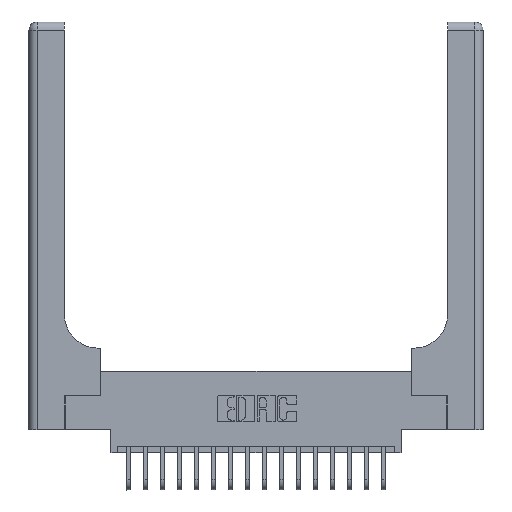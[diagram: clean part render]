
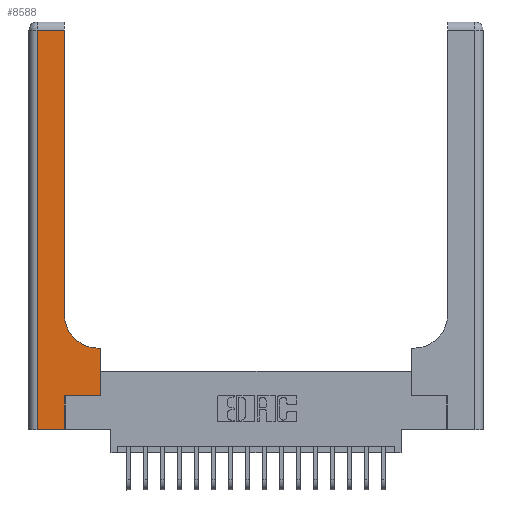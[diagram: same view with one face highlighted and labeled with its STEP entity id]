
A CAD part, top view. The second image highlights one B-rep face of the part: STEP entity #8588.
In plain terms, the highlighted planar face has unit normal (0, 0, 1).
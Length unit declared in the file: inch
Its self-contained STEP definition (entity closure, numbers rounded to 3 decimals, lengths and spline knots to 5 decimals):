
#76 = DIRECTION ( 'NONE',  ( 1., 0., 0. ) ) ;
#202 = EDGE_LOOP ( 'NONE', ( #3198, #1127, #1689, #18911, #7406, #10585, #1963, #21030, #20210 ) ) ;
#544 = VERTEX_POINT ( 'NONE', #6140 ) ;
#554 = DIRECTION ( 'NONE',  ( 1., 0., 0. ) ) ;
#799 = FACE_OUTER_BOUND ( 'NONE', #202, .T. ) ;
#1127 = ORIENTED_EDGE ( 'NONE', *, *, #20029, .T. ) ;
#1205 = AXIS2_PLACEMENT_3D ( 'NONE', #17898, #9666, #76 ) ;
#1557 = VECTOR ( 'NONE', #20072, 39.37008 ) ;
#1689 = ORIENTED_EDGE ( 'NONE', *, *, #18613, .T. ) ;
#1963 = ORIENTED_EDGE ( 'NONE', *, *, #7899, .T. ) ;
#1978 = LINE ( 'NONE', #5490, #5737 ) ;
#2013 = LINE ( 'NONE', #16639, #17235 ) ;
#2168 = CARTESIAN_POINT ( 'NONE',  ( 0.06, 3., 0.37 ) ) ;
#2465 = VERTEX_POINT ( 'NONE', #7567 ) ;
#2975 = EDGE_CURVE ( 'NONE', #14000, #4491, #12141, .T. ) ;
#3198 = ORIENTED_EDGE ( 'NONE', *, *, #15015, .T. ) ;
#3808 = DIRECTION ( 'NONE',  ( 0., 0., -1. ) ) ;
#4002 = CARTESIAN_POINT ( 'NONE',  ( 0.265, 0.25, 0.37 ) ) ;
#4491 = VERTEX_POINT ( 'NONE', #15877 ) ;
#4868 = CARTESIAN_POINT ( 'NONE',  ( 0.26, 3., 0.37 ) ) ;
#5490 = CARTESIAN_POINT ( 'NONE',  ( 0., 0., 0.37 ) ) ;
#5499 = PLANE ( 'NONE',  #17982 ) ;
#5737 = VECTOR ( 'NONE', #554, 39.37008 ) ;
#5819 = LINE ( 'NONE', #2168, #1557 ) ;
#5963 = VERTEX_POINT ( 'NONE', #4002 ) ;
#6140 = CARTESIAN_POINT ( 'NONE',  ( 0.265, 0., 0.37 ) ) ;
#6759 = LINE ( 'NONE', #4868, #17689 ) ;
#7202 = EDGE_CURVE ( 'NONE', #5963, #15020, #19916, .T. ) ;
#7406 = ORIENTED_EDGE ( 'NONE', *, *, #10179, .T. ) ;
#7567 = CARTESIAN_POINT ( 'NONE',  ( 0.06, 2.94, 0.37 ) ) ;
#7899 = EDGE_CURVE ( 'NONE', #15020, #15990, #14054, .T. ) ;
#8588 = ADVANCED_FACE ( 'NONE', ( #799 ), #5499, .F. ) ;
#8613 = DIRECTION ( 'NONE',  ( 0., 1., 0. ) ) ;
#9108 = DIRECTION ( 'NONE',  ( -1., 0., 0. ) ) ;
#9666 = DIRECTION ( 'NONE',  ( 0., 0., -1. ) ) ;
#10179 = EDGE_CURVE ( 'NONE', #544, #5963, #2013, .T. ) ;
#10470 = CARTESIAN_POINT ( 'NONE',  ( 0.26, 0.6, 0.37 ) ) ;
#10585 = ORIENTED_EDGE ( 'NONE', *, *, #7202, .T. ) ;
#11302 = VERTEX_POINT ( 'NONE', #16238 ) ;
#11448 = VERTEX_POINT ( 'NONE', #14975 ) ;
#12141 = CIRCLE ( 'NONE', #1205, 0.25 ) ;
#13337 = DIRECTION ( 'NONE',  ( 1., 0., 0. ) ) ;
#13431 = DIRECTION ( 'NONE',  ( -1., 0., 0. ) ) ;
#14000 = VERTEX_POINT ( 'NONE', #20704 ) ;
#14054 = LINE ( 'NONE', #18211, #17338 ) ;
#14759 = EDGE_CURVE ( 'NONE', #11448, #544, #1978, .T. ) ;
#14785 = DIRECTION ( 'NONE',  ( 0., 1., 0. ) ) ;
#14975 = CARTESIAN_POINT ( 'NONE',  ( 0.06, 0., 0.37 ) ) ;
#14979 = LINE ( 'NONE', #15945, #15987 ) ;
#15015 = EDGE_CURVE ( 'NONE', #4491, #11302, #6759, .T. ) ;
#15020 = VERTEX_POINT ( 'NONE', #16269 ) ;
#15657 = CARTESIAN_POINT ( 'NONE',  ( 0.528, 0.6, 0.37 ) ) ;
#15844 = EDGE_CURVE ( 'NONE', #15990, #14000, #18954, .T. ) ;
#15877 = CARTESIAN_POINT ( 'NONE',  ( 0.26, 0.85, 0.37 ) ) ;
#15945 = CARTESIAN_POINT ( 'NONE',  ( 0., 2.94, 0.37 ) ) ;
#15987 = VECTOR ( 'NONE', #17642, 39.37008 ) ;
#15990 = VERTEX_POINT ( 'NONE', #15657 ) ;
#16136 = VECTOR ( 'NONE', #9108, 39.37008 ) ;
#16238 = CARTESIAN_POINT ( 'NONE',  ( 0.26, 2.94, 0.37 ) ) ;
#16269 = CARTESIAN_POINT ( 'NONE',  ( 0.528, 0.25, 0.37 ) ) ;
#16510 = CARTESIAN_POINT ( 'NONE',  ( 0.265, 0.25, 0.37 ) ) ;
#16639 = CARTESIAN_POINT ( 'NONE',  ( 0.265, 0., 0.37 ) ) ;
#17235 = VECTOR ( 'NONE', #8613, 39.37008 ) ;
#17338 = VECTOR ( 'NONE', #18284, 39.37008 ) ;
#17642 = DIRECTION ( 'NONE',  ( -1., 0., 0. ) ) ;
#17689 = VECTOR ( 'NONE', #14785, 39.37008 ) ;
#17898 = CARTESIAN_POINT ( 'NONE',  ( 0.51, 0.85, 0.37 ) ) ;
#17982 = AXIS2_PLACEMENT_3D ( 'NONE', #18257, #3808, #13431 ) ;
#18211 = CARTESIAN_POINT ( 'NONE',  ( 0.528, 0.25, 0.37 ) ) ;
#18257 = CARTESIAN_POINT ( 'NONE',  ( 0., 3., 0.37 ) ) ;
#18284 = DIRECTION ( 'NONE',  ( 0., 1., 0. ) ) ;
#18613 = EDGE_CURVE ( 'NONE', #2465, #11448, #5819, .T. ) ;
#18911 = ORIENTED_EDGE ( 'NONE', *, *, #14759, .T. ) ;
#18954 = LINE ( 'NONE', #10470, #16136 ) ;
#19391 = VECTOR ( 'NONE', #13337, 39.37008 ) ;
#19916 = LINE ( 'NONE', #16510, #19391 ) ;
#20029 = EDGE_CURVE ( 'NONE', #11302, #2465, #14979, .T. ) ;
#20072 = DIRECTION ( 'NONE',  ( 0., -1., 0. ) ) ;
#20210 = ORIENTED_EDGE ( 'NONE', *, *, #2975, .T. ) ;
#20704 = CARTESIAN_POINT ( 'NONE',  ( 0.51, 0.6, 0.37 ) ) ;
#21030 = ORIENTED_EDGE ( 'NONE', *, *, #15844, .T. ) ;
